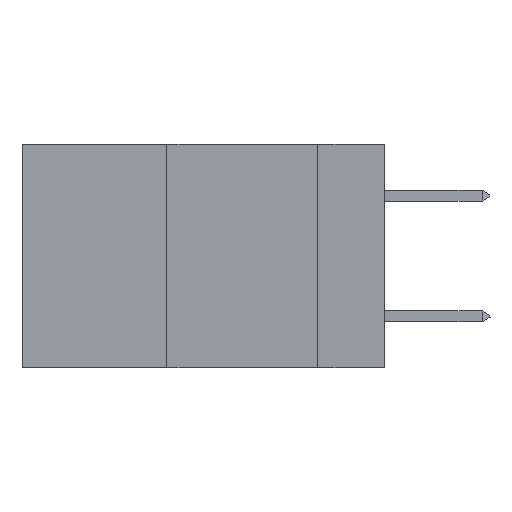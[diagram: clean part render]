
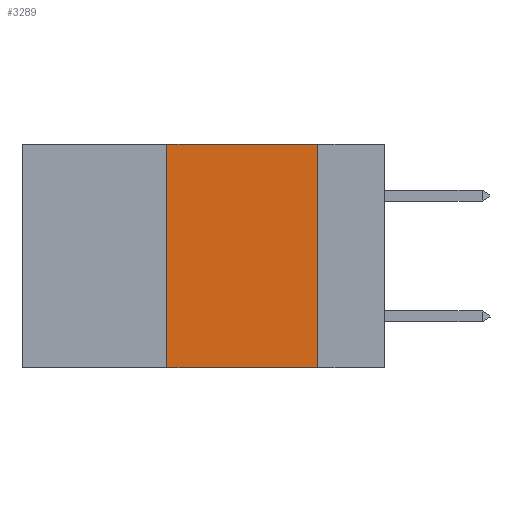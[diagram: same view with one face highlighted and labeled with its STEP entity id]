
A CAD part, left-side view. The second image highlights one B-rep face of the part: STEP entity #3289.
In plain terms, the highlighted planar face has unit normal (-1, 0, 0).
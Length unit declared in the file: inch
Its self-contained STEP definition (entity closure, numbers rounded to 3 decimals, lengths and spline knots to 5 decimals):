
#2664 = DIRECTION ( 'NONE',  ( 0., 0., -1. ) ) ;
#2844 = VERTEX_POINT ( 'NONE', #25842 ) ;
#2898 = DIRECTION ( 'NONE',  ( 0., 0., 1. ) ) ;
#3289 = ADVANCED_FACE ( 'NONE', ( #26418 ), #22981, .F. ) ;
#4230 = EDGE_CURVE ( 'NONE', #12414, #2844, #16820, .T. ) ;
#6347 = DIRECTION ( 'NONE',  ( 0., -1., 0. ) ) ;
#6485 = VECTOR ( 'NONE', #9220, 39.37008 ) ;
#7677 = CARTESIAN_POINT ( 'NONE',  ( 0., 0.11, 0. ) ) ;
#8346 = CARTESIAN_POINT ( 'NONE',  ( 0., 0.6, 0. ) ) ;
#8678 = CARTESIAN_POINT ( 'NONE',  ( 0., 0.36, 0. ) ) ;
#9173 = ORIENTED_EDGE ( 'NONE', *, *, #12176, .T. ) ;
#9220 = DIRECTION ( 'NONE',  ( 0., -1., 0. ) ) ;
#10784 = VECTOR ( 'NONE', #11045, 39.37008 ) ;
#10888 = LINE ( 'NONE', #8346, #28615 ) ;
#11045 = DIRECTION ( 'NONE',  ( 0., 0., -1. ) ) ;
#11570 = EDGE_CURVE ( 'NONE', #29028, #27136, #17818, .T. ) ;
#12176 = EDGE_CURVE ( 'NONE', #29028, #2844, #17104, .T. ) ;
#12414 = VERTEX_POINT ( 'NONE', #19401 ) ;
#13593 = VECTOR ( 'NONE', #2898, 39.37008 ) ;
#13976 = DIRECTION ( 'NONE',  ( 1., 0., 0. ) ) ;
#16820 = LINE ( 'NONE', #7677, #10784 ) ;
#17104 = LINE ( 'NONE', #22999, #6485 ) ;
#17818 = LINE ( 'NONE', #21231, #13593 ) ;
#19401 = CARTESIAN_POINT ( 'NONE',  ( 0., 0.11, 0. ) ) ;
#19575 = ORIENTED_EDGE ( 'NONE', *, *, #11570, .F. ) ;
#19907 = AXIS2_PLACEMENT_3D ( 'NONE', #23075, #13976, #2664 ) ;
#20742 = ORIENTED_EDGE ( 'NONE', *, *, #4230, .F. ) ;
#21231 = CARTESIAN_POINT ( 'NONE',  ( 0., 0.36, 0. ) ) ;
#22920 = EDGE_LOOP ( 'NONE', ( #20742, #26627, #19575, #9173 ) ) ;
#22981 = PLANE ( 'NONE',  #19907 ) ;
#22999 = CARTESIAN_POINT ( 'NONE',  ( 0., 0.6, -0.37 ) ) ;
#23075 = CARTESIAN_POINT ( 'NONE',  ( 0., 0.6, 0. ) ) ;
#23264 = CARTESIAN_POINT ( 'NONE',  ( 0., 0.36, -0.37 ) ) ;
#25842 = CARTESIAN_POINT ( 'NONE',  ( 0., 0.11, -0.37 ) ) ;
#26418 = FACE_OUTER_BOUND ( 'NONE', #22920, .T. ) ;
#26627 = ORIENTED_EDGE ( 'NONE', *, *, #28816, .F. ) ;
#27136 = VERTEX_POINT ( 'NONE', #8678 ) ;
#28615 = VECTOR ( 'NONE', #6347, 39.37008 ) ;
#28816 = EDGE_CURVE ( 'NONE', #27136, #12414, #10888, .T. ) ;
#29028 = VERTEX_POINT ( 'NONE', #23264 ) ;
